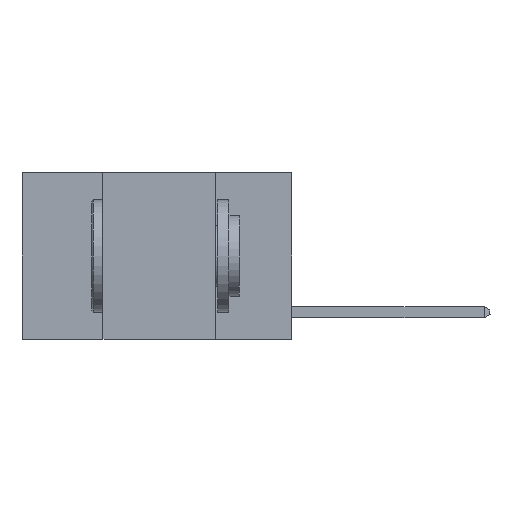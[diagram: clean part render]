
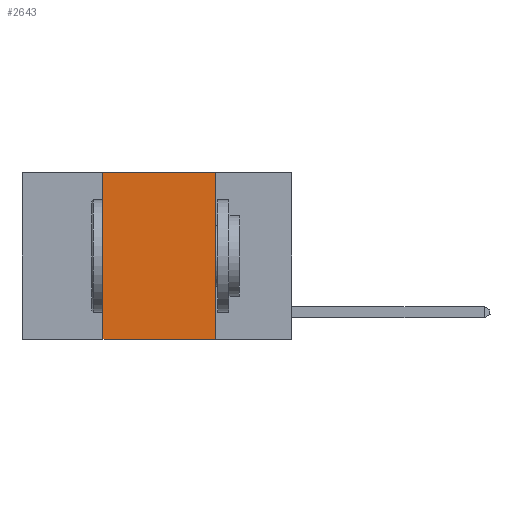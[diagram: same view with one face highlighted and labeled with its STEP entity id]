
A CAD part, left-side view. The second image highlights one B-rep face of the part: STEP entity #2643.
In plain terms, the highlighted planar face has unit normal (-1, 0, 0).
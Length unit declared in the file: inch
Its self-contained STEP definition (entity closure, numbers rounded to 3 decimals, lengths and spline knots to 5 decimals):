
#379 = VECTOR ( 'NONE', #7904, 39.37008 ) ;
#697 = EDGE_CURVE ( 'NONE', #1701, #8165, #5669, .T. ) ;
#1045 = ORIENTED_EDGE ( 'NONE', *, *, #697, .F. ) ;
#1062 = ORIENTED_EDGE ( 'NONE', *, *, #13051, .F. ) ;
#1087 = EDGE_LOOP ( 'NONE', ( #1062, #1045, #3607, #5371 ) ) ;
#1434 = CARTESIAN_POINT ( 'NONE',  ( 0., 0.42, 0. ) ) ;
#1701 = VERTEX_POINT ( 'NONE', #14024 ) ;
#2110 = CARTESIAN_POINT ( 'NONE',  ( 0., 0.42, -0.37 ) ) ;
#2312 = VECTOR ( 'NONE', #4787, 39.37008 ) ;
#2643 = ADVANCED_FACE ( 'NONE', ( #5098 ), #9483, .F. ) ;
#2859 = CARTESIAN_POINT ( 'NONE',  ( 0., 0.17, 0. ) ) ;
#3607 = ORIENTED_EDGE ( 'NONE', *, *, #12301, .F. ) ;
#4074 = AXIS2_PLACEMENT_3D ( 'NONE', #10210, #5185, #9888 ) ;
#4351 = LINE ( 'NONE', #2859, #10187 ) ;
#4787 = DIRECTION ( 'NONE',  ( 0., 0., 1. ) ) ;
#5098 = FACE_OUTER_BOUND ( 'NONE', #1087, .T. ) ;
#5185 = DIRECTION ( 'NONE',  ( 1., 0., 0. ) ) ;
#5195 = EDGE_CURVE ( 'NONE', #13321, #7671, #6239, .T. ) ;
#5371 = ORIENTED_EDGE ( 'NONE', *, *, #5195, .T. ) ;
#5669 = LINE ( 'NONE', #9535, #14098 ) ;
#6239 = LINE ( 'NONE', #12382, #379 ) ;
#7671 = VERTEX_POINT ( 'NONE', #10315 ) ;
#7904 = DIRECTION ( 'NONE',  ( 0., -1., 0. ) ) ;
#8165 = VERTEX_POINT ( 'NONE', #10196 ) ;
#9483 = PLANE ( 'NONE',  #4074 ) ;
#9535 = CARTESIAN_POINT ( 'NONE',  ( 0., 0.6, 0. ) ) ;
#9888 = DIRECTION ( 'NONE',  ( 0., 0., -1. ) ) ;
#10187 = VECTOR ( 'NONE', #10542, 39.37008 ) ;
#10196 = CARTESIAN_POINT ( 'NONE',  ( 0., 0.17, 0. ) ) ;
#10210 = CARTESIAN_POINT ( 'NONE',  ( 0., 0.6, 0. ) ) ;
#10315 = CARTESIAN_POINT ( 'NONE',  ( 0., 0.17, -0.37 ) ) ;
#10542 = DIRECTION ( 'NONE',  ( 0., 0., -1. ) ) ;
#10885 = DIRECTION ( 'NONE',  ( 0., -1., 0. ) ) ;
#12301 = EDGE_CURVE ( 'NONE', #13321, #1701, #14000, .T. ) ;
#12382 = CARTESIAN_POINT ( 'NONE',  ( 0., 0.6, -0.37 ) ) ;
#13051 = EDGE_CURVE ( 'NONE', #8165, #7671, #4351, .T. ) ;
#13321 = VERTEX_POINT ( 'NONE', #2110 ) ;
#14000 = LINE ( 'NONE', #1434, #2312 ) ;
#14024 = CARTESIAN_POINT ( 'NONE',  ( 0., 0.42, 0. ) ) ;
#14098 = VECTOR ( 'NONE', #10885, 39.37008 ) ;
